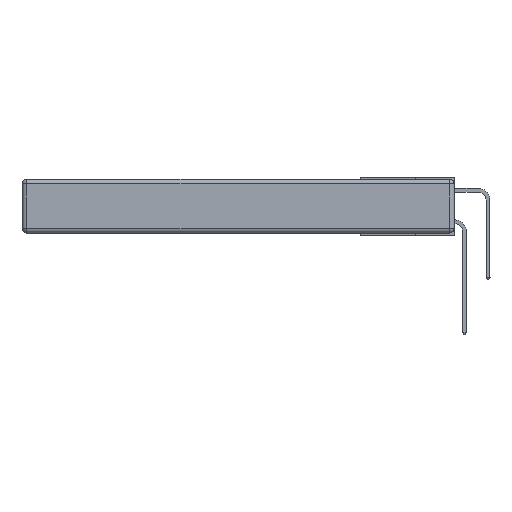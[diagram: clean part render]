
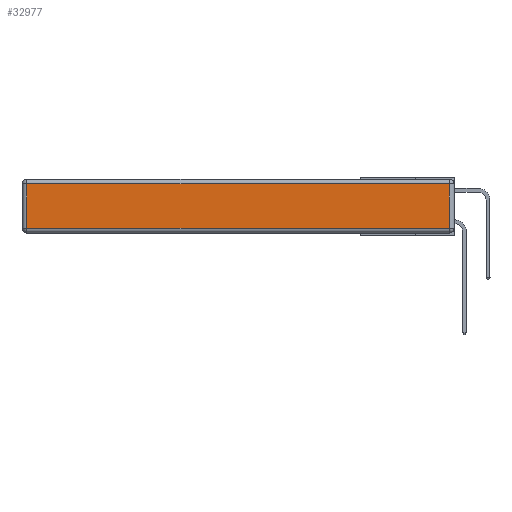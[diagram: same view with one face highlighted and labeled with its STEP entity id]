
A CAD part, left-side view. The second image highlights one B-rep face of the part: STEP entity #32977.
In plain terms, the highlighted planar face has unit normal (-1, 0, 0).
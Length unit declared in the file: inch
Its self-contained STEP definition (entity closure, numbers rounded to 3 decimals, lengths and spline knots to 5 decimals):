
#306 = CARTESIAN_POINT ( 'NONE',  ( 0., 0., -0.313 ) ) ;
#2399 = EDGE_LOOP ( 'NONE', ( #28755, #6532, #33665, #18964 ) ) ;
#3241 = VECTOR ( 'NONE', #24218, 39.37008 ) ;
#5749 = CARTESIAN_POINT ( 'NONE',  ( 0., 0.03, -0.343 ) ) ;
#6197 = CARTESIAN_POINT ( 'NONE',  ( 0., 2.72, -0.313 ) ) ;
#6532 = ORIENTED_EDGE ( 'NONE', *, *, #28292, .T. ) ;
#8648 = CARTESIAN_POINT ( 'NONE',  ( 0., 0.03, -0.313 ) ) ;
#8886 = VECTOR ( 'NONE', #24031, 39.37008 ) ;
#9456 = VERTEX_POINT ( 'NONE', #15173 ) ;
#11261 = DIRECTION ( 'NONE',  ( 0., 1., 0. ) ) ;
#12864 = DIRECTION ( 'NONE',  ( -1., 0., 0. ) ) ;
#14169 = DIRECTION ( 'NONE',  ( 0., -1., 0. ) ) ;
#14249 = VECTOR ( 'NONE', #11261, 39.37008 ) ;
#14482 = EDGE_CURVE ( 'NONE', #32107, #14521, #23870, .T. ) ;
#14521 = VERTEX_POINT ( 'NONE', #8648 ) ;
#14698 = LINE ( 'NONE', #24102, #3241 ) ;
#15173 = CARTESIAN_POINT ( 'NONE',  ( 0., 0.03, -0.03 ) ) ;
#15383 = VERTEX_POINT ( 'NONE', #22830 ) ;
#15505 = DIRECTION ( 'NONE',  ( 0., 0., 1. ) ) ;
#15901 = LINE ( 'NONE', #31765, #14249 ) ;
#15978 = AXIS2_PLACEMENT_3D ( 'NONE', #28745, #12864, #15505 ) ;
#17818 = PLANE ( 'NONE',  #15978 ) ;
#18964 = ORIENTED_EDGE ( 'NONE', *, *, #31488, .T. ) ;
#22830 = CARTESIAN_POINT ( 'NONE',  ( 0., 2.72, -0.03 ) ) ;
#23057 = VECTOR ( 'NONE', #14169, 39.37008 ) ;
#23870 = LINE ( 'NONE', #306, #23057 ) ;
#24031 = DIRECTION ( 'NONE',  ( 0., 0., 1. ) ) ;
#24102 = CARTESIAN_POINT ( 'NONE',  ( 0., 2.72, -0.343 ) ) ;
#24218 = DIRECTION ( 'NONE',  ( 0., 0., -1. ) ) ;
#27311 = FACE_OUTER_BOUND ( 'NONE', #2399, .T. ) ;
#27920 = EDGE_CURVE ( 'NONE', #9456, #15383, #15901, .T. ) ;
#28292 = EDGE_CURVE ( 'NONE', #14521, #9456, #28952, .T. ) ;
#28745 = CARTESIAN_POINT ( 'NONE',  ( 0., 0., -0.343 ) ) ;
#28755 = ORIENTED_EDGE ( 'NONE', *, *, #14482, .T. ) ;
#28952 = LINE ( 'NONE', #5749, #8886 ) ;
#31488 = EDGE_CURVE ( 'NONE', #15383, #32107, #14698, .T. ) ;
#31765 = CARTESIAN_POINT ( 'NONE',  ( 0., 2.75, -0.03 ) ) ;
#32107 = VERTEX_POINT ( 'NONE', #6197 ) ;
#32977 = ADVANCED_FACE ( 'NONE', ( #27311 ), #17818, .T. ) ;
#33665 = ORIENTED_EDGE ( 'NONE', *, *, #27920, .T. ) ;
